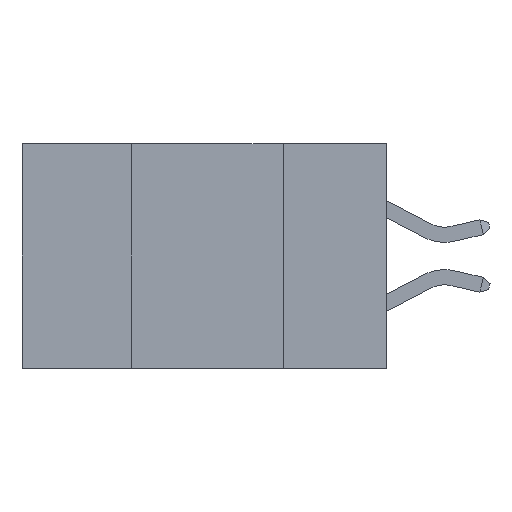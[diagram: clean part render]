
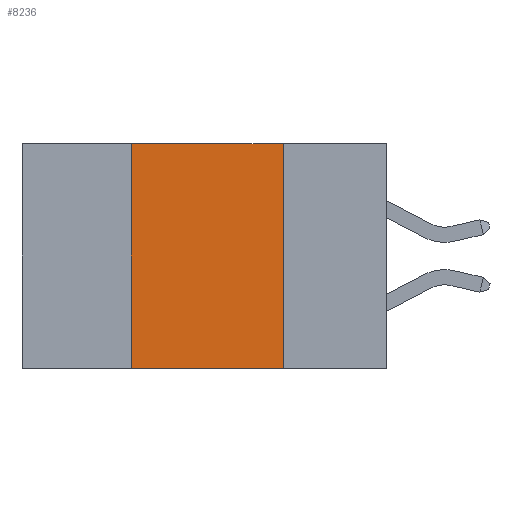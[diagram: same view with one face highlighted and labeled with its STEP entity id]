
A CAD part, left-side view. The second image highlights one B-rep face of the part: STEP entity #8236.
In plain terms, the highlighted planar face has unit normal (-1, 0, 0).
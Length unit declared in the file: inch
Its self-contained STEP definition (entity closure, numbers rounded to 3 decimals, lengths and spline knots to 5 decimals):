
#891 = LINE ( 'NONE', #8517, #6991 ) ;
#1228 = DIRECTION ( 'NONE',  ( 0., 0., -1. ) ) ;
#1959 = CARTESIAN_POINT ( 'NONE',  ( 0., 0.42, 0. ) ) ;
#2208 = LINE ( 'NONE', #10400, #6627 ) ;
#2700 = VECTOR ( 'NONE', #13171, 39.37008 ) ;
#2894 = CARTESIAN_POINT ( 'NONE',  ( 0., 0.17, -0.37 ) ) ;
#2950 = EDGE_CURVE ( 'NONE', #7917, #13036, #5505, .T. ) ;
#3744 = ORIENTED_EDGE ( 'NONE', *, *, #3949, .T. ) ;
#3949 = EDGE_CURVE ( 'NONE', #7917, #8121, #2208, .T. ) ;
#3998 = DIRECTION ( 'NONE',  ( 1., 0., 0. ) ) ;
#4126 = EDGE_CURVE ( 'NONE', #13036, #4666, #10863, .T. ) ;
#4420 = DIRECTION ( 'NONE',  ( 0., -1., 0. ) ) ;
#4666 = VERTEX_POINT ( 'NONE', #5420 ) ;
#5420 = CARTESIAN_POINT ( 'NONE',  ( 0., 0.17, 0. ) ) ;
#5505 = LINE ( 'NONE', #9994, #2700 ) ;
#6627 = VECTOR ( 'NONE', #8338, 39.37008 ) ;
#6991 = VECTOR ( 'NONE', #1228, 39.37008 ) ;
#7917 = VERTEX_POINT ( 'NONE', #9973 ) ;
#8121 = VERTEX_POINT ( 'NONE', #2894 ) ;
#8236 = ADVANCED_FACE ( 'NONE', ( #10072 ), #11226, .F. ) ;
#8338 = DIRECTION ( 'NONE',  ( 0., -1., 0. ) ) ;
#8517 = CARTESIAN_POINT ( 'NONE',  ( 0., 0.17, 0. ) ) ;
#8879 = VECTOR ( 'NONE', #4420, 39.37008 ) ;
#9973 = CARTESIAN_POINT ( 'NONE',  ( 0., 0.42, -0.37 ) ) ;
#9994 = CARTESIAN_POINT ( 'NONE',  ( 0., 0.42, 0. ) ) ;
#10072 = FACE_OUTER_BOUND ( 'NONE', #12752, .T. ) ;
#10287 = CARTESIAN_POINT ( 'NONE',  ( 0., 0.6, 0. ) ) ;
#10400 = CARTESIAN_POINT ( 'NONE',  ( 0., 0.6, -0.37 ) ) ;
#10404 = ORIENTED_EDGE ( 'NONE', *, *, #12050, .F. ) ;
#10670 = CARTESIAN_POINT ( 'NONE',  ( 0., 0.6, 0. ) ) ;
#10863 = LINE ( 'NONE', #10670, #8879 ) ;
#11117 = ORIENTED_EDGE ( 'NONE', *, *, #4126, .F. ) ;
#11226 = PLANE ( 'NONE',  #13149 ) ;
#11416 = ORIENTED_EDGE ( 'NONE', *, *, #2950, .F. ) ;
#12050 = EDGE_CURVE ( 'NONE', #4666, #8121, #891, .T. ) ;
#12382 = DIRECTION ( 'NONE',  ( 0., 0., -1. ) ) ;
#12752 = EDGE_LOOP ( 'NONE', ( #10404, #11117, #11416, #3744 ) ) ;
#13036 = VERTEX_POINT ( 'NONE', #1959 ) ;
#13149 = AXIS2_PLACEMENT_3D ( 'NONE', #10287, #3998, #12382 ) ;
#13171 = DIRECTION ( 'NONE',  ( 0., 0., 1. ) ) ;
